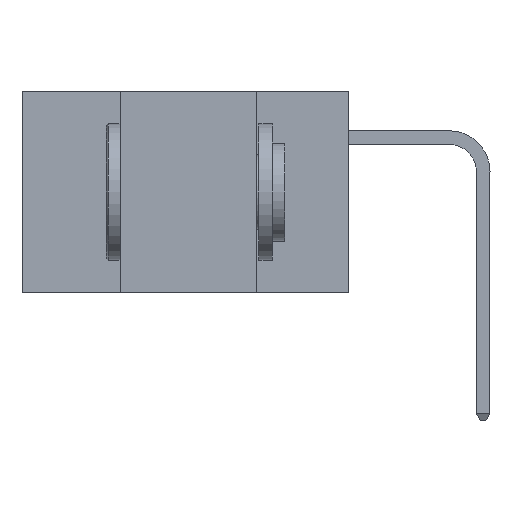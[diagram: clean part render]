
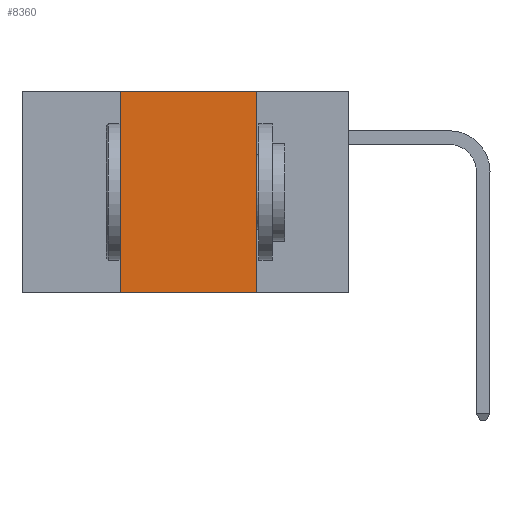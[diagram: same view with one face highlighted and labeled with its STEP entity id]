
A CAD part, left-side view. The second image highlights one B-rep face of the part: STEP entity #8360.
In plain terms, the highlighted planar face has unit normal (-1, 0, 0).
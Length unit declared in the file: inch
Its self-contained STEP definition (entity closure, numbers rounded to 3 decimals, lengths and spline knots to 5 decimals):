
#1257 = VERTEX_POINT ( 'NONE', #22418 ) ;
#1708 = CARTESIAN_POINT ( 'NONE',  ( 0., 0.42, 0. ) ) ;
#1798 = EDGE_CURVE ( 'NONE', #1257, #9849, #3288, .T. ) ;
#1959 = VERTEX_POINT ( 'NONE', #3014 ) ;
#2007 = FACE_OUTER_BOUND ( 'NONE', #20144, .T. ) ;
#2507 = DIRECTION ( 'NONE',  ( 0., 0., -1. ) ) ;
#3014 = CARTESIAN_POINT ( 'NONE',  ( 0., 0.42, 0. ) ) ;
#3288 = LINE ( 'NONE', #11992, #22792 ) ;
#3697 = DIRECTION ( 'NONE',  ( 0., 0., 1. ) ) ;
#4596 = EDGE_CURVE ( 'NONE', #1257, #1959, #8408, .T. ) ;
#6242 = PLANE ( 'NONE',  #7884 ) ;
#7351 = VECTOR ( 'NONE', #20686, 39.37008 ) ;
#7884 = AXIS2_PLACEMENT_3D ( 'NONE', #23260, #19485, #8152 ) ;
#8152 = DIRECTION ( 'NONE',  ( 0., 0., -1. ) ) ;
#8360 = ADVANCED_FACE ( 'NONE', ( #2007 ), #6242, .F. ) ;
#8408 = LINE ( 'NONE', #1708, #19060 ) ;
#9849 = VERTEX_POINT ( 'NONE', #12099 ) ;
#11841 = VECTOR ( 'NONE', #2507, 39.37008 ) ;
#11992 = CARTESIAN_POINT ( 'NONE',  ( 0., 0.6, -0.37 ) ) ;
#12099 = CARTESIAN_POINT ( 'NONE',  ( 0., 0.17, -0.37 ) ) ;
#12120 = EDGE_CURVE ( 'NONE', #1959, #16039, #20679, .T. ) ;
#13696 = ORIENTED_EDGE ( 'NONE', *, *, #17499, .F. ) ;
#15608 = ORIENTED_EDGE ( 'NONE', *, *, #12120, .F. ) ;
#15838 = ORIENTED_EDGE ( 'NONE', *, *, #1798, .T. ) ;
#16039 = VERTEX_POINT ( 'NONE', #22426 ) ;
#16162 = CARTESIAN_POINT ( 'NONE',  ( 0., 0.6, 0. ) ) ;
#17499 = EDGE_CURVE ( 'NONE', #16039, #9849, #18322, .T. ) ;
#17812 = ORIENTED_EDGE ( 'NONE', *, *, #4596, .F. ) ;
#18322 = LINE ( 'NONE', #19445, #11841 ) ;
#19060 = VECTOR ( 'NONE', #3697, 39.37008 ) ;
#19445 = CARTESIAN_POINT ( 'NONE',  ( 0., 0.17, 0. ) ) ;
#19485 = DIRECTION ( 'NONE',  ( 1., 0., 0. ) ) ;
#20144 = EDGE_LOOP ( 'NONE', ( #13696, #15608, #17812, #15838 ) ) ;
#20679 = LINE ( 'NONE', #16162, #7351 ) ;
#20686 = DIRECTION ( 'NONE',  ( 0., -1., 0. ) ) ;
#21116 = DIRECTION ( 'NONE',  ( 0., -1., 0. ) ) ;
#22418 = CARTESIAN_POINT ( 'NONE',  ( 0., 0.42, -0.37 ) ) ;
#22426 = CARTESIAN_POINT ( 'NONE',  ( 0., 0.17, 0. ) ) ;
#22792 = VECTOR ( 'NONE', #21116, 39.37008 ) ;
#23260 = CARTESIAN_POINT ( 'NONE',  ( 0., 0.6, 0. ) ) ;
